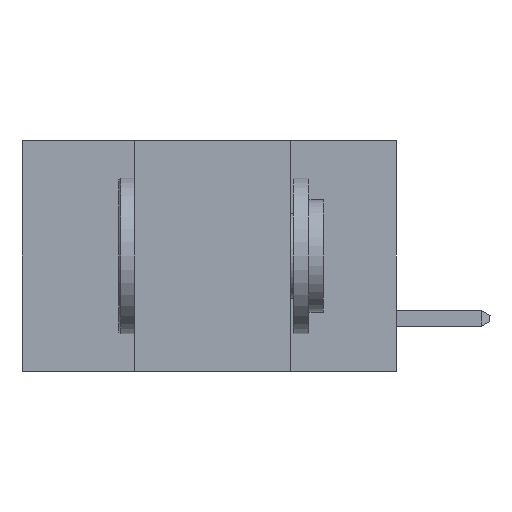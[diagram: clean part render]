
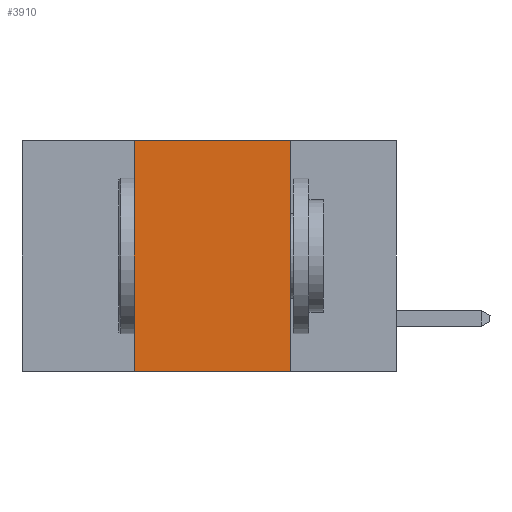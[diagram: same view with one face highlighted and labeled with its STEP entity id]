
A CAD part, left-side view. The second image highlights one B-rep face of the part: STEP entity #3910.
In plain terms, the highlighted planar face has unit normal (-1, 0, 0).
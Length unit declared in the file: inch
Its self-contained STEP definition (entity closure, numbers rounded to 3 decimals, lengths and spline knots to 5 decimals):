
#164 = LINE ( 'NONE', #4387, #6201 ) ;
#375 = AXIS2_PLACEMENT_3D ( 'NONE', #786, #1366, #811 ) ;
#452 = VECTOR ( 'NONE', #2757, 39.37008 ) ;
#712 = ORIENTED_EDGE ( 'NONE', *, *, #4611, .F. ) ;
#786 = CARTESIAN_POINT ( 'NONE',  ( 0., 0.6, 0. ) ) ;
#811 = DIRECTION ( 'NONE',  ( 0., 0., -1. ) ) ;
#1246 = DIRECTION ( 'NONE',  ( 0., 0., -1. ) ) ;
#1366 = DIRECTION ( 'NONE',  ( 1., 0., 0. ) ) ;
#1399 = DIRECTION ( 'NONE',  ( 0., -1., 0. ) ) ;
#1463 = LINE ( 'NONE', #6914, #2595 ) ;
#1524 = PLANE ( 'NONE',  #375 ) ;
#2595 = VECTOR ( 'NONE', #1246, 39.37008 ) ;
#2605 = VERTEX_POINT ( 'NONE', #8171 ) ;
#2757 = DIRECTION ( 'NONE',  ( 0., -1., 0. ) ) ;
#2771 = FACE_OUTER_BOUND ( 'NONE', #9196, .T. ) ;
#3140 = LINE ( 'NONE', #7808, #5306 ) ;
#3435 = ORIENTED_EDGE ( 'NONE', *, *, #4081, .T. ) ;
#3752 = VERTEX_POINT ( 'NONE', #4567 ) ;
#3910 = ADVANCED_FACE ( 'NONE', ( #2771 ), #1524, .F. ) ;
#4081 = EDGE_CURVE ( 'NONE', #3752, #5145, #4824, .T. ) ;
#4387 = CARTESIAN_POINT ( 'NONE',  ( 0., 0.42, -0.37 ) ) ;
#4567 = CARTESIAN_POINT ( 'NONE',  ( 0., 0.42, -0.37 ) ) ;
#4611 = EDGE_CURVE ( 'NONE', #3752, #2605, #164, .T. ) ;
#4824 = LINE ( 'NONE', #8968, #452 ) ;
#5145 = VERTEX_POINT ( 'NONE', #5839 ) ;
#5186 = DIRECTION ( 'NONE',  ( 0., 0., 1. ) ) ;
#5306 = VECTOR ( 'NONE', #1399, 39.37008 ) ;
#5839 = CARTESIAN_POINT ( 'NONE',  ( 0., 0.17, -0.37 ) ) ;
#6201 = VECTOR ( 'NONE', #5186, 39.37008 ) ;
#6235 = EDGE_CURVE ( 'NONE', #2605, #9243, #3140, .T. ) ;
#6579 = ORIENTED_EDGE ( 'NONE', *, *, #6745, .F. ) ;
#6745 = EDGE_CURVE ( 'NONE', #9243, #5145, #1463, .T. ) ;
#6914 = CARTESIAN_POINT ( 'NONE',  ( 0., 0.17, -0.37 ) ) ;
#7505 = CARTESIAN_POINT ( 'NONE',  ( 0., 0.17, 0. ) ) ;
#7808 = CARTESIAN_POINT ( 'NONE',  ( 0., 0.6, 0. ) ) ;
#8171 = CARTESIAN_POINT ( 'NONE',  ( 0., 0.42, 0. ) ) ;
#8968 = CARTESIAN_POINT ( 'NONE',  ( 0., 0.6, -0.37 ) ) ;
#9179 = ORIENTED_EDGE ( 'NONE', *, *, #6235, .F. ) ;
#9196 = EDGE_LOOP ( 'NONE', ( #6579, #9179, #712, #3435 ) ) ;
#9243 = VERTEX_POINT ( 'NONE', #7505 ) ;
